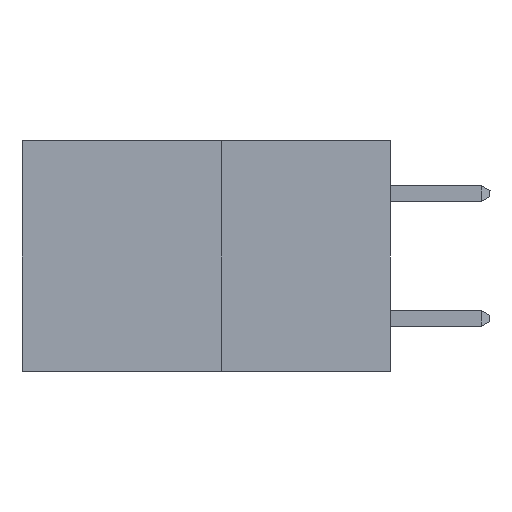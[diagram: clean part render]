
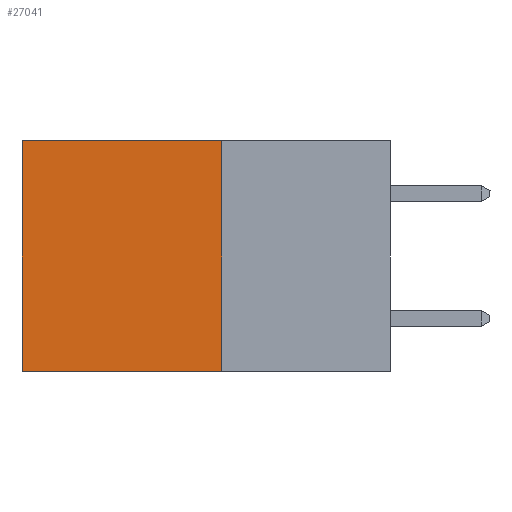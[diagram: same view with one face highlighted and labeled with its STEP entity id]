
A CAD part, left-side view. The second image highlights one B-rep face of the part: STEP entity #27041.
In plain terms, the highlighted planar face has unit normal (-1, 0, 0).
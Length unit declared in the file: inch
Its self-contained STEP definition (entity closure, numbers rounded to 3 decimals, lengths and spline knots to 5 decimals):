
#704 = ORIENTED_EDGE ( 'NONE', *, *, #24171, .T. ) ;
#1401 = CARTESIAN_POINT ( 'NONE',  ( 0.277, 0.27, -0.37 ) ) ;
#3254 = VERTEX_POINT ( 'NONE', #1401 ) ;
#3333 = CARTESIAN_POINT ( 'NONE',  ( 0.277, 0.27, -0.37 ) ) ;
#3572 = ORIENTED_EDGE ( 'NONE', *, *, #25899, .F. ) ;
#4728 = PLANE ( 'NONE',  #12289 ) ;
#6509 = LINE ( 'NONE', #11401, #27837 ) ;
#6703 = LINE ( 'NONE', #19054, #24277 ) ;
#6944 = CARTESIAN_POINT ( 'NONE',  ( 0.277, 0.27, -0.37 ) ) ;
#7978 = VECTOR ( 'NONE', #28284, 39.37008 ) ;
#8388 = CARTESIAN_POINT ( 'NONE',  ( 0.277, 0.59, -0.37 ) ) ;
#9149 = DIRECTION ( 'NONE',  ( 1., 0., 0. ) ) ;
#11401 = CARTESIAN_POINT ( 'NONE',  ( 0.277, 0.27, -0.37 ) ) ;
#11983 = FACE_OUTER_BOUND ( 'NONE', #13240, .T. ) ;
#12289 = AXIS2_PLACEMENT_3D ( 'NONE', #6944, #9149, #24556 ) ;
#13189 = ORIENTED_EDGE ( 'NONE', *, *, #21637, .F. ) ;
#13240 = EDGE_LOOP ( 'NONE', ( #704, #3572, #13189, #20092 ) ) ;
#14275 = DIRECTION ( 'NONE',  ( 0., 1., 0. ) ) ;
#16783 = VECTOR ( 'NONE', #14275, 39.37008 ) ;
#16791 = CARTESIAN_POINT ( 'NONE',  ( 0.277, 0.59, 0. ) ) ;
#17106 = VERTEX_POINT ( 'NONE', #16791 ) ;
#17484 = LINE ( 'NONE', #3333, #16783 ) ;
#17556 = VERTEX_POINT ( 'NONE', #27039 ) ;
#18463 = EDGE_CURVE ( 'NONE', #22577, #17106, #6703, .T. ) ;
#19054 = CARTESIAN_POINT ( 'NONE',  ( 0.277, 0.27, 0. ) ) ;
#20092 = ORIENTED_EDGE ( 'NONE', *, *, #18463, .T. ) ;
#20295 = LINE ( 'NONE', #8388, #7978 ) ;
#20729 = CARTESIAN_POINT ( 'NONE',  ( 0.277, 0.27, 0. ) ) ;
#21270 = DIRECTION ( 'NONE',  ( 0., 1., 0. ) ) ;
#21637 = EDGE_CURVE ( 'NONE', #22577, #3254, #6509, .T. ) ;
#22577 = VERTEX_POINT ( 'NONE', #20729 ) ;
#24171 = EDGE_CURVE ( 'NONE', #17106, #17556, #20295, .T. ) ;
#24277 = VECTOR ( 'NONE', #21270, 39.37008 ) ;
#24556 = DIRECTION ( 'NONE',  ( 0., 0., -1. ) ) ;
#25899 = EDGE_CURVE ( 'NONE', #3254, #17556, #17484, .T. ) ;
#26791 = DIRECTION ( 'NONE',  ( 0., 0., -1. ) ) ;
#27039 = CARTESIAN_POINT ( 'NONE',  ( 0.277, 0.59, -0.37 ) ) ;
#27041 = ADVANCED_FACE ( 'NONE', ( #11983 ), #4728, .F. ) ;
#27837 = VECTOR ( 'NONE', #26791, 39.37008 ) ;
#28284 = DIRECTION ( 'NONE',  ( 0., 0., -1. ) ) ;
